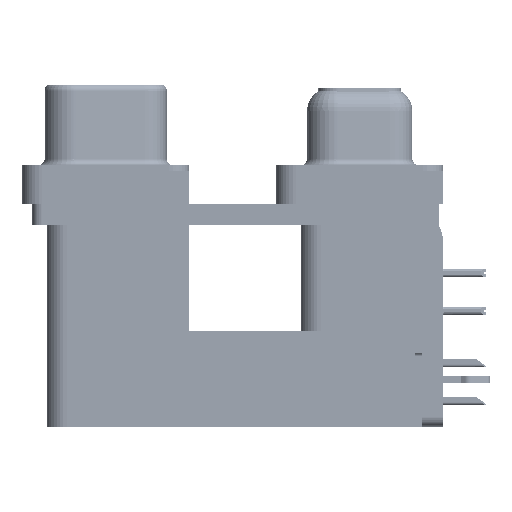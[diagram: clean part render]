
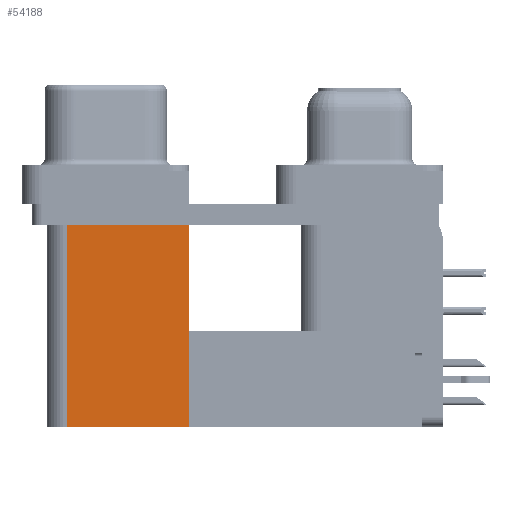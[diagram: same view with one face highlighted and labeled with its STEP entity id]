
A CAD part, left-side view. The second image highlights one B-rep face of the part: STEP entity #54188.
In plain terms, the highlighted planar face has unit normal (-1, 0, 0).
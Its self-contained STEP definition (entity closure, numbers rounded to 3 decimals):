
#982 = CARTESIAN_POINT ( 'NONE',  ( 3.7, 21.975, -2.5 ) ) ;
#1229 = ORIENTED_EDGE ( 'NONE', *, *, #32462, .F. ) ;
#1521 = VERTEX_POINT ( 'NONE', #982 ) ;
#2008 = EDGE_CURVE ( 'NONE', #7350, #2300, #39704, .T. ) ;
#2300 = VERTEX_POINT ( 'NONE', #51744 ) ;
#2992 = CARTESIAN_POINT ( 'NONE',  ( 3.7, 21.975, -19.2 ) ) ;
#3742 = DIRECTION ( 'NONE',  ( 0., 1., 0. ) ) ;
#4572 = CARTESIAN_POINT ( 'NONE',  ( 3.7, 12.775, -19.2 ) ) ;
#7029 = VERTEX_POINT ( 'NONE', #33210 ) ;
#7350 = VERTEX_POINT ( 'NONE', #15358 ) ;
#8952 = DIRECTION ( 'NONE',  ( 0., 0., 1. ) ) ;
#10271 = EDGE_LOOP ( 'NONE', ( #39247, #1229, #28572, #26297 ) ) ;
#13080 = DIRECTION ( 'NONE',  ( 0., 1., 0. ) ) ;
#13138 = VECTOR ( 'NONE', #20501, 1000. ) ;
#15358 = CARTESIAN_POINT ( 'NONE',  ( 3.7, 12.775, -19.2 ) ) ;
#17143 = DIRECTION ( 'NONE',  ( 0., 1., 0. ) ) ;
#18227 = LINE ( 'NONE', #48159, #44583 ) ;
#20501 = DIRECTION ( 'NONE',  ( 0., 0., 1. ) ) ;
#26118 = FACE_OUTER_BOUND ( 'NONE', #10271, .T. ) ;
#26297 = ORIENTED_EDGE ( 'NONE', *, *, #2008, .T. ) ;
#28572 = ORIENTED_EDGE ( 'NONE', *, *, #47067, .F. ) ;
#32462 = EDGE_CURVE ( 'NONE', #7029, #1521, #46683, .T. ) ;
#33210 = CARTESIAN_POINT ( 'NONE',  ( 3.7, 21.975, -19.2 ) ) ;
#35324 = EDGE_CURVE ( 'NONE', #2300, #1521, #18227, .T. ) ;
#36419 = VECTOR ( 'NONE', #17143, 1000. ) ;
#39247 = ORIENTED_EDGE ( 'NONE', *, *, #35324, .T. ) ;
#39704 = LINE ( 'NONE', #44602, #46212 ) ;
#41506 = AXIS2_PLACEMENT_3D ( 'NONE', #4572, #48824, #3742 ) ;
#43952 = PLANE ( 'NONE',  #41506 ) ;
#44583 = VECTOR ( 'NONE', #13080, 1000. ) ;
#44602 = CARTESIAN_POINT ( 'NONE',  ( 3.7, 12.775, -19.2 ) ) ;
#46212 = VECTOR ( 'NONE', #8952, 1000. ) ;
#46683 = LINE ( 'NONE', #2992, #13138 ) ;
#47067 = EDGE_CURVE ( 'NONE', #7350, #7029, #51639, .T. ) ;
#47616 = CARTESIAN_POINT ( 'NONE',  ( 3.7, 12.775, -19.2 ) ) ;
#48159 = CARTESIAN_POINT ( 'NONE',  ( 3.7, 12.775, -2.5 ) ) ;
#48824 = DIRECTION ( 'NONE',  ( 1., 0., 0. ) ) ;
#51639 = LINE ( 'NONE', #47616, #36419 ) ;
#51744 = CARTESIAN_POINT ( 'NONE',  ( 3.7, 12.775, -2.5 ) ) ;
#54188 = ADVANCED_FACE ( 'NONE', ( #26118 ), #43952, .F. ) ;
